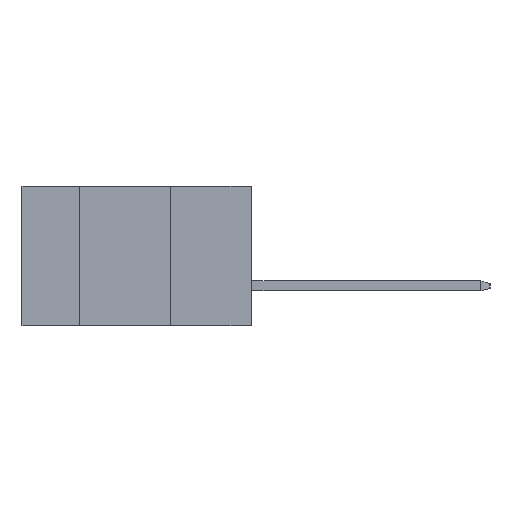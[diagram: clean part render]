
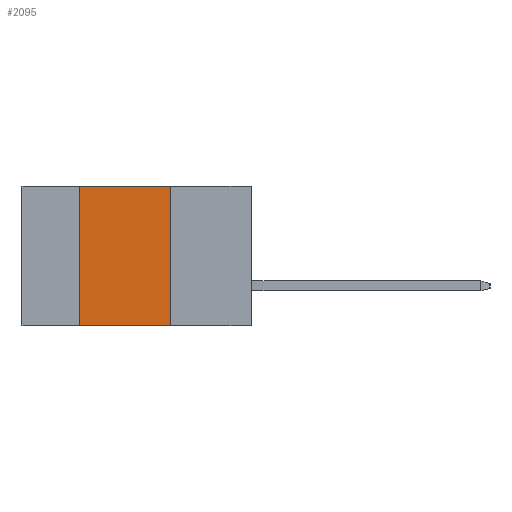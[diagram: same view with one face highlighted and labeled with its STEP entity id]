
A CAD part, left-side view. The second image highlights one B-rep face of the part: STEP entity #2095.
In plain terms, the highlighted planar face has unit normal (-1, 0, 0).
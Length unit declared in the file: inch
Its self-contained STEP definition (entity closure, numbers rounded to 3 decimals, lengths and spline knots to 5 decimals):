
#1312 = DIRECTION ( 'NONE',  ( 1., 0., 0. ) ) ;
#1633 = DIRECTION ( 'NONE',  ( 0., -1., 0. ) ) ;
#1801 = EDGE_CURVE ( 'NONE', #4617, #8823, #5248, .T. ) ;
#2095 = ADVANCED_FACE ( 'NONE', ( #2189 ), #5709, .F. ) ;
#2189 = FACE_OUTER_BOUND ( 'NONE', #3878, .T. ) ;
#2421 = CARTESIAN_POINT ( 'NONE',  ( 0., 0.54, 0. ) ) ;
#2561 = DIRECTION ( 'NONE',  ( 0., 0., -1. ) ) ;
#2762 = LINE ( 'NONE', #8056, #10474 ) ;
#3346 = VERTEX_POINT ( 'NONE', #3809 ) ;
#3735 = VECTOR ( 'NONE', #2561, 39.37008 ) ;
#3744 = CARTESIAN_POINT ( 'NONE',  ( 0., 0.54, -0.437 ) ) ;
#3809 = CARTESIAN_POINT ( 'NONE',  ( 0., 0.254, -0.437 ) ) ;
#3878 = EDGE_LOOP ( 'NONE', ( #10924, #10860, #9884, #9768 ) ) ;
#4343 = EDGE_CURVE ( 'NONE', #10191, #3346, #7803, .T. ) ;
#4617 = VERTEX_POINT ( 'NONE', #9692 ) ;
#4791 = VECTOR ( 'NONE', #7896, 39.37008 ) ;
#4844 = DIRECTION ( 'NONE',  ( 0., 0., -1. ) ) ;
#5144 = CARTESIAN_POINT ( 'NONE',  ( 0., 0.254, 0. ) ) ;
#5248 = LINE ( 'NONE', #3744, #4791 ) ;
#5709 = PLANE ( 'NONE',  #5724 ) ;
#5724 = AXIS2_PLACEMENT_3D ( 'NONE', #9213, #1312, #4844 ) ;
#6211 = CARTESIAN_POINT ( 'NONE',  ( 0., 0.72, 0. ) ) ;
#6296 = DIRECTION ( 'NONE',  ( 0., -1., 0. ) ) ;
#7037 = EDGE_CURVE ( 'NONE', #8823, #10191, #10582, .T. ) ;
#7168 = CARTESIAN_POINT ( 'NONE',  ( 0., 0.254, -0.437 ) ) ;
#7803 = LINE ( 'NONE', #7168, #3735 ) ;
#7896 = DIRECTION ( 'NONE',  ( 0., 0., 1. ) ) ;
#8056 = CARTESIAN_POINT ( 'NONE',  ( 0., 0.72, -0.437 ) ) ;
#8823 = VERTEX_POINT ( 'NONE', #2421 ) ;
#9213 = CARTESIAN_POINT ( 'NONE',  ( 0., 0.72, 0. ) ) ;
#9692 = CARTESIAN_POINT ( 'NONE',  ( 0., 0.54, -0.437 ) ) ;
#9768 = ORIENTED_EDGE ( 'NONE', *, *, #10702, .T. ) ;
#9884 = ORIENTED_EDGE ( 'NONE', *, *, #1801, .F. ) ;
#10191 = VERTEX_POINT ( 'NONE', #5144 ) ;
#10474 = VECTOR ( 'NONE', #6296, 39.37008 ) ;
#10582 = LINE ( 'NONE', #6211, #10618 ) ;
#10618 = VECTOR ( 'NONE', #1633, 39.37008 ) ;
#10702 = EDGE_CURVE ( 'NONE', #4617, #3346, #2762, .T. ) ;
#10860 = ORIENTED_EDGE ( 'NONE', *, *, #7037, .F. ) ;
#10924 = ORIENTED_EDGE ( 'NONE', *, *, #4343, .F. ) ;
